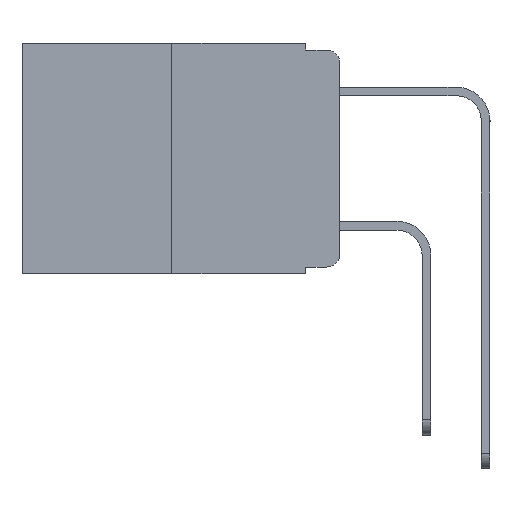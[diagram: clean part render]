
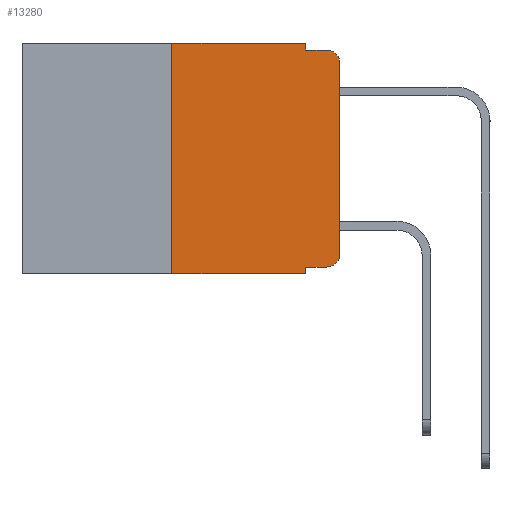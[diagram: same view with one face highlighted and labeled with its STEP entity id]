
A CAD part, left-side view. The second image highlights one B-rep face of the part: STEP entity #13280.
In plain terms, the highlighted planar face has unit normal (-1, 0, 0).
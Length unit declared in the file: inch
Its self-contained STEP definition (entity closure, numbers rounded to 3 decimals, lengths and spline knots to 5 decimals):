
#19 = ORIENTED_EDGE ( 'NONE', *, *, #10527, .F. ) ;
#69 = VERTEX_POINT ( 'NONE', #11155 ) ;
#411 = LINE ( 'NONE', #10823, #14611 ) ;
#649 = DIRECTION ( 'NONE',  ( 1., 0., 0. ) ) ;
#912 = VERTEX_POINT ( 'NONE', #8601 ) ;
#1144 = ORIENTED_EDGE ( 'NONE', *, *, #9359, .F. ) ;
#1699 = CARTESIAN_POINT ( 'NONE',  ( 0., 0.051, 0. ) ) ;
#1900 = VERTEX_POINT ( 'NONE', #8758 ) ;
#2250 = AXIS2_PLACEMENT_3D ( 'NONE', #19122, #8602, #20855 ) ;
#2251 = CARTESIAN_POINT ( 'NONE',  ( 0., 0.051, -0.333 ) ) ;
#2372 = VECTOR ( 'NONE', #4789, 39.37008 ) ;
#2936 = LINE ( 'NONE', #18879, #2372 ) ;
#3142 = DIRECTION ( 'NONE',  ( -1., 0., 0. ) ) ;
#3388 = EDGE_CURVE ( 'NONE', #14686, #4029, #14317, .T. ) ;
#3690 = DIRECTION ( 'NONE',  ( 0., -1., 0. ) ) ;
#3709 = EDGE_CURVE ( 'NONE', #9857, #5336, #12079, .T. ) ;
#4029 = VERTEX_POINT ( 'NONE', #9545 ) ;
#4086 = CARTESIAN_POINT ( 'NONE',  ( 0., 0.051, -0.333 ) ) ;
#4423 = CARTESIAN_POINT ( 'NONE',  ( 0., 0., 0. ) ) ;
#4601 = EDGE_CURVE ( 'NONE', #8817, #14686, #10100, .T. ) ;
#4789 = DIRECTION ( 'NONE',  ( 0., -1., 0. ) ) ;
#5182 = VECTOR ( 'NONE', #15995, 39.37008 ) ;
#5336 = VERTEX_POINT ( 'NONE', #15534 ) ;
#5355 = VECTOR ( 'NONE', #3690, 39.37008 ) ;
#5370 = AXIS2_PLACEMENT_3D ( 'NONE', #13766, #3142, #12073 ) ;
#5778 = EDGE_CURVE ( 'NONE', #8817, #5336, #17999, .T. ) ;
#6185 = CIRCLE ( 'NONE', #2250, 0.02 ) ;
#6306 = CARTESIAN_POINT ( 'NONE',  ( 0., 0.25, -0.343 ) ) ;
#6677 = CARTESIAN_POINT ( 'NONE',  ( 0., 0.473, 0. ) ) ;
#7022 = ORIENTED_EDGE ( 'NONE', *, *, #8143, .F. ) ;
#7614 = VERTEX_POINT ( 'NONE', #12846 ) ;
#7748 = AXIS2_PLACEMENT_3D ( 'NONE', #11324, #649, #13092 ) ;
#8069 = VECTOR ( 'NONE', #17896, 39.37008 ) ;
#8117 = ORIENTED_EDGE ( 'NONE', *, *, #5778, .F. ) ;
#8143 = EDGE_CURVE ( 'NONE', #9857, #1900, #9928, .T. ) ;
#8601 = CARTESIAN_POINT ( 'NONE',  ( 0., 0.051, 0. ) ) ;
#8602 = DIRECTION ( 'NONE',  ( -1., 0., 0. ) ) ;
#8758 = CARTESIAN_POINT ( 'NONE',  ( 0., 0.25, 0. ) ) ;
#8817 = VERTEX_POINT ( 'NONE', #2251 ) ;
#9358 = CARTESIAN_POINT ( 'NONE',  ( 0., 0.02, -0.333 ) ) ;
#9359 = EDGE_CURVE ( 'NONE', #912, #11441, #411, .T. ) ;
#9545 = CARTESIAN_POINT ( 'NONE',  ( 0., 0., -0.313 ) ) ;
#9857 = VERTEX_POINT ( 'NONE', #6306 ) ;
#9928 = LINE ( 'NONE', #14213, #5182 ) ;
#9971 = EDGE_CURVE ( 'NONE', #1900, #912, #11024, .T. ) ;
#10100 = LINE ( 'NONE', #4086, #5355 ) ;
#10459 = VECTOR ( 'NONE', #18980, 39.37008 ) ;
#10527 = EDGE_CURVE ( 'NONE', #11441, #69, #2936, .T. ) ;
#10823 = CARTESIAN_POINT ( 'NONE',  ( 0., 0.051, 0. ) ) ;
#11024 = LINE ( 'NONE', #6677, #10459 ) ;
#11155 = CARTESIAN_POINT ( 'NONE',  ( 0., 0.02, -0.01 ) ) ;
#11324 = CARTESIAN_POINT ( 'NONE',  ( 0., 0.473, 0. ) ) ;
#11441 = VERTEX_POINT ( 'NONE', #15415 ) ;
#11454 = ORIENTED_EDGE ( 'NONE', *, *, #12909, .T. ) ;
#12073 = DIRECTION ( 'NONE',  ( 0., 0., -1. ) ) ;
#12079 = LINE ( 'NONE', #16715, #20799 ) ;
#12846 = CARTESIAN_POINT ( 'NONE',  ( 0., 0., -0.03 ) ) ;
#12909 = EDGE_CURVE ( 'NONE', #7614, #69, #6185, .T. ) ;
#13092 = DIRECTION ( 'NONE',  ( 0., 0., -1. ) ) ;
#13280 = ADVANCED_FACE ( 'NONE', ( #18296 ), #21751, .F. ) ;
#13766 = CARTESIAN_POINT ( 'NONE',  ( 0., 0.02, -0.313 ) ) ;
#13947 = ORIENTED_EDGE ( 'NONE', *, *, #4601, .T. ) ;
#14086 = EDGE_CURVE ( 'NONE', #4029, #7614, #14735, .T. ) ;
#14213 = CARTESIAN_POINT ( 'NONE',  ( 0., 0.25, 0. ) ) ;
#14317 = CIRCLE ( 'NONE', #5370, 0.02 ) ;
#14611 = VECTOR ( 'NONE', #21286, 39.37008 ) ;
#14686 = VERTEX_POINT ( 'NONE', #9358 ) ;
#14735 = LINE ( 'NONE', #4423, #15302 ) ;
#15054 = DIRECTION ( 'NONE',  ( 0., 0., 1. ) ) ;
#15302 = VECTOR ( 'NONE', #15054, 39.37008 ) ;
#15415 = CARTESIAN_POINT ( 'NONE',  ( 0., 0.051, -0.01 ) ) ;
#15534 = CARTESIAN_POINT ( 'NONE',  ( 0., 0.051, -0.343 ) ) ;
#15882 = ORIENTED_EDGE ( 'NONE', *, *, #9971, .F. ) ;
#15995 = DIRECTION ( 'NONE',  ( 0., 0., 1. ) ) ;
#16715 = CARTESIAN_POINT ( 'NONE',  ( 0., 0.473, -0.343 ) ) ;
#17500 = EDGE_LOOP ( 'NONE', ( #19102, #11454, #19, #1144, #15882, #7022, #21545, #8117, #13947, #20222 ) ) ;
#17896 = DIRECTION ( 'NONE',  ( 0., 0., -1. ) ) ;
#17999 = LINE ( 'NONE', #1699, #8069 ) ;
#18296 = FACE_OUTER_BOUND ( 'NONE', #17500, .T. ) ;
#18879 = CARTESIAN_POINT ( 'NONE',  ( 0., 0.051, -0.01 ) ) ;
#18980 = DIRECTION ( 'NONE',  ( 0., -1., 0. ) ) ;
#19102 = ORIENTED_EDGE ( 'NONE', *, *, #14086, .T. ) ;
#19122 = CARTESIAN_POINT ( 'NONE',  ( 0., 0.02, -0.03 ) ) ;
#20222 = ORIENTED_EDGE ( 'NONE', *, *, #3388, .T. ) ;
#20799 = VECTOR ( 'NONE', #20823, 39.37008 ) ;
#20823 = DIRECTION ( 'NONE',  ( 0., -1., 0. ) ) ;
#20855 = DIRECTION ( 'NONE',  ( 0., 0., -1. ) ) ;
#21286 = DIRECTION ( 'NONE',  ( 0., 0., -1. ) ) ;
#21545 = ORIENTED_EDGE ( 'NONE', *, *, #3709, .T. ) ;
#21751 = PLANE ( 'NONE',  #7748 ) ;
